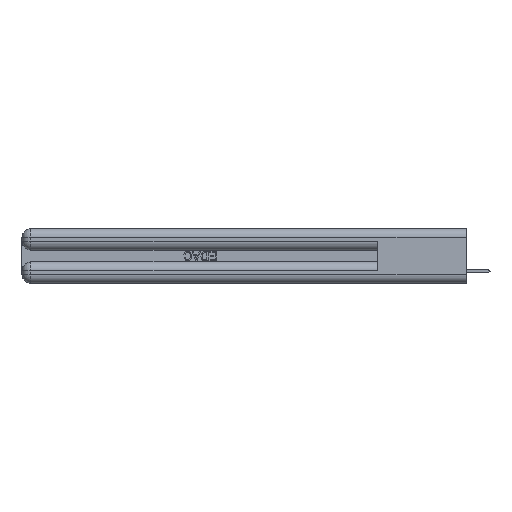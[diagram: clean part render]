
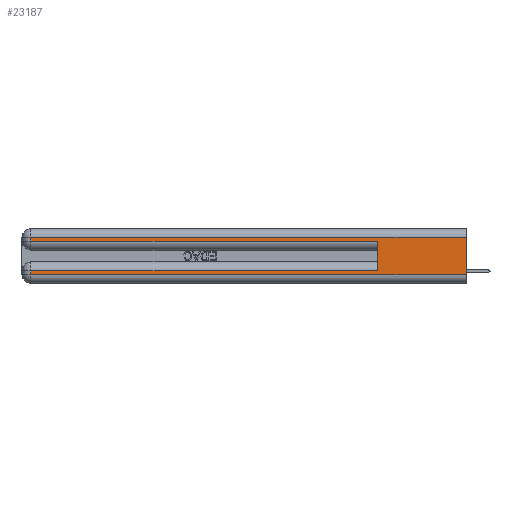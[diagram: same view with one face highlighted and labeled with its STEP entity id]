
A CAD part, left-side view. The second image highlights one B-rep face of the part: STEP entity #23187.
In plain terms, the highlighted planar face has unit normal (-1, 0, 0).
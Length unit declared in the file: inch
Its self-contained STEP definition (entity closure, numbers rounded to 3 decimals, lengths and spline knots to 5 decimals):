
#28 = VERTEX_POINT ( 'NONE', #21729 ) ;
#268 = ORIENTED_EDGE ( 'NONE', *, *, #24254, .T. ) ;
#797 = CARTESIAN_POINT ( 'NONE',  ( 0., 0.6, 0.085 ) ) ;
#1252 = DIRECTION ( 'NONE',  ( 0., 0., 1. ) ) ;
#2039 = CARTESIAN_POINT ( 'NONE',  ( 0., 0., 0.37 ) ) ;
#2453 = CARTESIAN_POINT ( 'NONE',  ( 0., 0., 0.285 ) ) ;
#2786 = CARTESIAN_POINT ( 'NONE',  ( 0., 2.94, 0.37 ) ) ;
#3444 = VECTOR ( 'NONE', #15395, 39.37008 ) ;
#5618 = CARTESIAN_POINT ( 'NONE',  ( 0., 0.6, 0.145 ) ) ;
#6287 = LINE ( 'NONE', #20091, #10229 ) ;
#6804 = ORIENTED_EDGE ( 'NONE', *, *, #46516, .T. ) ;
#7242 = LINE ( 'NONE', #35135, #49562 ) ;
#7501 = LINE ( 'NONE', #2453, #3444 ) ;
#9025 = LINE ( 'NONE', #2039, #32967 ) ;
#10229 = VECTOR ( 'NONE', #54525, 39.37008 ) ;
#10380 = ORIENTED_EDGE ( 'NONE', *, *, #46441, .T. ) ;
#10683 = CARTESIAN_POINT ( 'NONE',  ( 0., 0., 0.06 ) ) ;
#13718 = VECTOR ( 'NONE', #29846, 39.37008 ) ;
#14561 = DIRECTION ( 'NONE',  ( 1., 0., 0. ) ) ;
#14911 = EDGE_CURVE ( 'NONE', #20278, #52875, #9025, .T. ) ;
#15395 = DIRECTION ( 'NONE',  ( 0., -1., 0. ) ) ;
#16050 = ORIENTED_EDGE ( 'NONE', *, *, #14911, .F. ) ;
#16184 = AXIS2_PLACEMENT_3D ( 'NONE', #38459, #14561, #23104 ) ;
#20091 = CARTESIAN_POINT ( 'NONE',  ( 0., 0., 0.06 ) ) ;
#20278 = VERTEX_POINT ( 'NONE', #48196 ) ;
#20957 = VERTEX_POINT ( 'NONE', #53698 ) ;
#21729 = CARTESIAN_POINT ( 'NONE',  ( 0., 2.94, 0.285 ) ) ;
#22497 = ORIENTED_EDGE ( 'NONE', *, *, #27956, .T. ) ;
#22500 = EDGE_CURVE ( 'NONE', #33723, #23191, #40694, .T. ) ;
#23104 = DIRECTION ( 'NONE',  ( 0., 0., -1. ) ) ;
#23187 = ADVANCED_FACE ( 'NONE', ( #47161 ), #35215, .F. ) ;
#23191 = VERTEX_POINT ( 'NONE', #33697 ) ;
#24254 = EDGE_CURVE ( 'NONE', #28, #23191, #7501, .T. ) ;
#25667 = VECTOR ( 'NONE', #49601, 39.37008 ) ;
#26596 = CARTESIAN_POINT ( 'NONE',  ( 0., 2.94, 0.085 ) ) ;
#27766 = VERTEX_POINT ( 'NONE', #26596 ) ;
#27956 = EDGE_CURVE ( 'NONE', #20957, #52875, #6287, .T. ) ;
#28397 = LINE ( 'NONE', #50907, #13718 ) ;
#29846 = DIRECTION ( 'NONE',  ( 0., 1., 0. ) ) ;
#31604 = DIRECTION ( 'NONE',  ( 0., 0., -1. ) ) ;
#32882 = VECTOR ( 'NONE', #34117, 39.37008 ) ;
#32967 = VECTOR ( 'NONE', #31604, 39.37008 ) ;
#33697 = CARTESIAN_POINT ( 'NONE',  ( 0., 0.6, 0.285 ) ) ;
#33723 = VERTEX_POINT ( 'NONE', #797 ) ;
#34117 = DIRECTION ( 'NONE',  ( 0., 1., 0. ) ) ;
#34956 = DIRECTION ( 'NONE',  ( 0., 0., -1. ) ) ;
#35135 = CARTESIAN_POINT ( 'NONE',  ( 0., 2.94, 0.37 ) ) ;
#35215 = PLANE ( 'NONE',  #16184 ) ;
#36494 = ORIENTED_EDGE ( 'NONE', *, *, #22500, .F. ) ;
#38273 = LINE ( 'NONE', #2786, #25667 ) ;
#38459 = CARTESIAN_POINT ( 'NONE',  ( 0., 0., 0.37 ) ) ;
#38652 = CARTESIAN_POINT ( 'NONE',  ( 0., 0., 0.085 ) ) ;
#38666 = CARTESIAN_POINT ( 'NONE',  ( 0., 2.94, 0.31 ) ) ;
#38836 = ORIENTED_EDGE ( 'NONE', *, *, #52537, .T. ) ;
#40694 = LINE ( 'NONE', #5618, #45421 ) ;
#40745 = LINE ( 'NONE', #38652, #32882 ) ;
#44429 = EDGE_LOOP ( 'NONE', ( #16050, #10380, #50137, #268, #36494, #38836, #6804, #22497 ) ) ;
#45421 = VECTOR ( 'NONE', #1252, 39.37008 ) ;
#46441 = EDGE_CURVE ( 'NONE', #20278, #50796, #28397, .T. ) ;
#46516 = EDGE_CURVE ( 'NONE', #27766, #20957, #7242, .T. ) ;
#46823 = EDGE_CURVE ( 'NONE', #50796, #28, #38273, .T. ) ;
#47161 = FACE_OUTER_BOUND ( 'NONE', #44429, .T. ) ;
#48196 = CARTESIAN_POINT ( 'NONE',  ( 0., 0., 0.31 ) ) ;
#49562 = VECTOR ( 'NONE', #34956, 39.37008 ) ;
#49601 = DIRECTION ( 'NONE',  ( 0., 0., -1. ) ) ;
#50137 = ORIENTED_EDGE ( 'NONE', *, *, #46823, .T. ) ;
#50796 = VERTEX_POINT ( 'NONE', #38666 ) ;
#50907 = CARTESIAN_POINT ( 'NONE',  ( 0., 0., 0.31 ) ) ;
#52537 = EDGE_CURVE ( 'NONE', #33723, #27766, #40745, .T. ) ;
#52875 = VERTEX_POINT ( 'NONE', #10683 ) ;
#53698 = CARTESIAN_POINT ( 'NONE',  ( 0., 2.94, 0.06 ) ) ;
#54525 = DIRECTION ( 'NONE',  ( 0., -1., 0. ) ) ;
